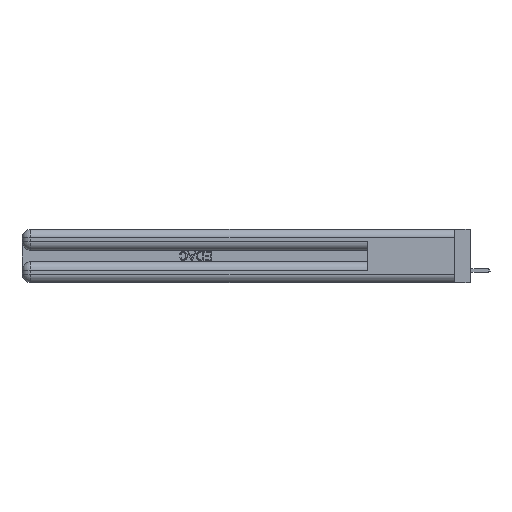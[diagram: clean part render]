
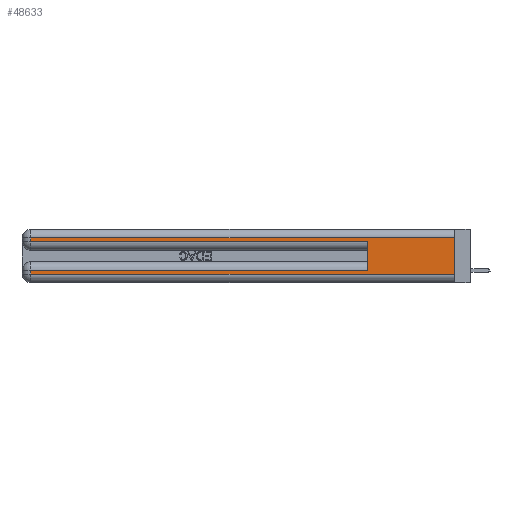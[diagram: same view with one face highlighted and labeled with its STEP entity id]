
A CAD part, left-side view. The second image highlights one B-rep face of the part: STEP entity #48633.
In plain terms, the highlighted planar face has unit normal (-1, 0, 0).
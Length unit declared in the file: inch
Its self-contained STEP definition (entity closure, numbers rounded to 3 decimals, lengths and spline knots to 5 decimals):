
#207 = LINE ( 'NONE', #12034, #20232 ) ;
#1550 = ORIENTED_EDGE ( 'NONE', *, *, #48693, .T. ) ;
#2845 = ORIENTED_EDGE ( 'NONE', *, *, #7062, .T. ) ;
#4514 = DIRECTION ( 'NONE',  ( 0., 0., -1. ) ) ;
#5003 = DIRECTION ( 'NONE',  ( 0., 1., 0. ) ) ;
#7062 = EDGE_CURVE ( 'NONE', #47290, #46892, #33783, .T. ) ;
#7433 = EDGE_CURVE ( 'NONE', #47290, #24325, #207, .T. ) ;
#7924 = LINE ( 'NONE', #43993, #45491 ) ;
#8159 = DIRECTION ( 'NONE',  ( 0., 0., -1. ) ) ;
#8420 = CARTESIAN_POINT ( 'NONE',  ( 0., 0., 0.31 ) ) ;
#8892 = EDGE_CURVE ( 'NONE', #46892, #20332, #15967, .T. ) ;
#10401 = VERTEX_POINT ( 'NONE', #18233 ) ;
#10686 = VECTOR ( 'NONE', #18576, 39.37008 ) ;
#10850 = ORIENTED_EDGE ( 'NONE', *, *, #19505, .F. ) ;
#11187 = CARTESIAN_POINT ( 'NONE',  ( 0., 2.94, 0.37 ) ) ;
#12034 = CARTESIAN_POINT ( 'NONE',  ( 0., 0., 0.37 ) ) ;
#12580 = DIRECTION ( 'NONE',  ( 0., 0., -1. ) ) ;
#15178 = DIRECTION ( 'NONE',  ( 0., 0., 1. ) ) ;
#15967 = LINE ( 'NONE', #11187, #30077 ) ;
#17963 = ORIENTED_EDGE ( 'NONE', *, *, #34388, .T. ) ;
#18233 = CARTESIAN_POINT ( 'NONE',  ( 0., 2.94, 0.06 ) ) ;
#18576 = DIRECTION ( 'NONE',  ( 0., -1., 0. ) ) ;
#19505 = EDGE_CURVE ( 'NONE', #43198, #28782, #30478, .T. ) ;
#20232 = VECTOR ( 'NONE', #8159, 39.37008 ) ;
#20304 = CARTESIAN_POINT ( 'NONE',  ( 0., 0., 0.085 ) ) ;
#20332 = VERTEX_POINT ( 'NONE', #31229 ) ;
#20486 = CARTESIAN_POINT ( 'NONE',  ( 0., 2.94, 0.31 ) ) ;
#22381 = ORIENTED_EDGE ( 'NONE', *, *, #35052, .T. ) ;
#22543 = CARTESIAN_POINT ( 'NONE',  ( 0., 0.6, 0.145 ) ) ;
#23510 = CARTESIAN_POINT ( 'NONE',  ( 0., 0., 0.31 ) ) ;
#23598 = LINE ( 'NONE', #20304, #28938 ) ;
#24325 = VERTEX_POINT ( 'NONE', #32468 ) ;
#24358 = VECTOR ( 'NONE', #41929, 39.37008 ) ;
#24701 = LINE ( 'NONE', #33800, #10686 ) ;
#28782 = VERTEX_POINT ( 'NONE', #44590 ) ;
#28938 = VECTOR ( 'NONE', #5003, 39.37008 ) ;
#30077 = VECTOR ( 'NONE', #4514, 39.37008 ) ;
#30478 = LINE ( 'NONE', #22543, #35208 ) ;
#31229 = CARTESIAN_POINT ( 'NONE',  ( 0., 2.94, 0.285 ) ) ;
#31454 = DIRECTION ( 'NONE',  ( 1., 0., 0. ) ) ;
#31788 = EDGE_CURVE ( 'NONE', #10401, #24325, #24701, .T. ) ;
#31957 = CARTESIAN_POINT ( 'NONE',  ( 0., 0., 0.37 ) ) ;
#32468 = CARTESIAN_POINT ( 'NONE',  ( 0., 0., 0.06 ) ) ;
#32791 = DIRECTION ( 'NONE',  ( 0., 0., -1. ) ) ;
#33243 = LINE ( 'NONE', #40485, #47978 ) ;
#33449 = ORIENTED_EDGE ( 'NONE', *, *, #8892, .T. ) ;
#33783 = LINE ( 'NONE', #8420, #24358 ) ;
#33800 = CARTESIAN_POINT ( 'NONE',  ( 0., 0., 0.06 ) ) ;
#34388 = EDGE_CURVE ( 'NONE', #20332, #28782, #33243, .T. ) ;
#35052 = EDGE_CURVE ( 'NONE', #37002, #10401, #7924, .T. ) ;
#35208 = VECTOR ( 'NONE', #15178, 39.37008 ) ;
#37002 = VERTEX_POINT ( 'NONE', #41493 ) ;
#39852 = AXIS2_PLACEMENT_3D ( 'NONE', #31957, #31454, #12580 ) ;
#40485 = CARTESIAN_POINT ( 'NONE',  ( 0., 0., 0.285 ) ) ;
#40689 = ORIENTED_EDGE ( 'NONE', *, *, #31788, .T. ) ;
#41088 = ORIENTED_EDGE ( 'NONE', *, *, #7433, .F. ) ;
#41413 = EDGE_LOOP ( 'NONE', ( #41088, #2845, #33449, #17963, #10850, #1550, #22381, #40689 ) ) ;
#41493 = CARTESIAN_POINT ( 'NONE',  ( 0., 2.94, 0.085 ) ) ;
#41929 = DIRECTION ( 'NONE',  ( 0., 1., 0. ) ) ;
#42980 = FACE_OUTER_BOUND ( 'NONE', #41413, .T. ) ;
#43198 = VERTEX_POINT ( 'NONE', #44864 ) ;
#43993 = CARTESIAN_POINT ( 'NONE',  ( 0., 2.94, 0.37 ) ) ;
#44404 = DIRECTION ( 'NONE',  ( 0., -1., 0. ) ) ;
#44590 = CARTESIAN_POINT ( 'NONE',  ( 0., 0.6, 0.285 ) ) ;
#44864 = CARTESIAN_POINT ( 'NONE',  ( 0., 0.6, 0.085 ) ) ;
#45491 = VECTOR ( 'NONE', #32791, 39.37008 ) ;
#46892 = VERTEX_POINT ( 'NONE', #20486 ) ;
#46915 = PLANE ( 'NONE',  #39852 ) ;
#47290 = VERTEX_POINT ( 'NONE', #23510 ) ;
#47978 = VECTOR ( 'NONE', #44404, 39.37008 ) ;
#48633 = ADVANCED_FACE ( 'NONE', ( #42980 ), #46915, .F. ) ;
#48693 = EDGE_CURVE ( 'NONE', #43198, #37002, #23598, .T. ) ;
